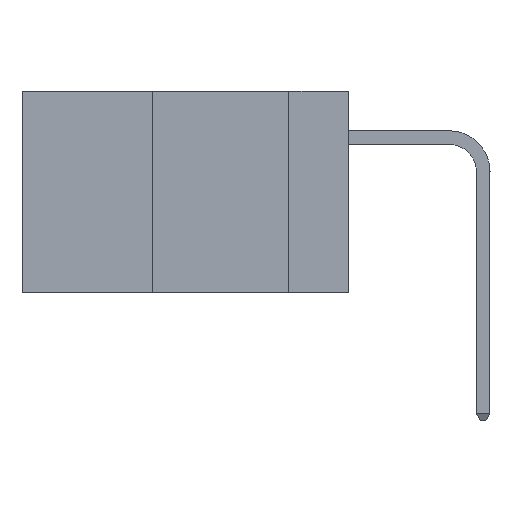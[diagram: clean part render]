
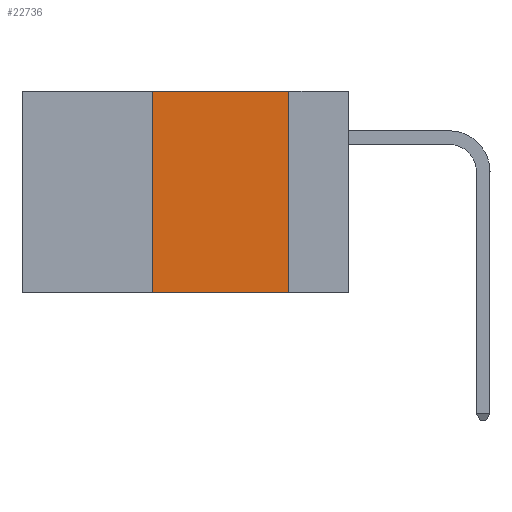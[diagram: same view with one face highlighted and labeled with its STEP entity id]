
A CAD part, left-side view. The second image highlights one B-rep face of the part: STEP entity #22736.
In plain terms, the highlighted planar face has unit normal (-1, 0, 0).
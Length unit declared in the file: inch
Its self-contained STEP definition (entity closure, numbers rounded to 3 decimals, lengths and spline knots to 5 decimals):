
#1048 = CARTESIAN_POINT ( 'NONE',  ( 0., 0.11, 0. ) ) ;
#1820 = VERTEX_POINT ( 'NONE', #23831 ) ;
#2241 = VECTOR ( 'NONE', #38119, 39.37008 ) ;
#2506 = CARTESIAN_POINT ( 'NONE',  ( 0., 0.36, 0. ) ) ;
#2942 = DIRECTION ( 'NONE',  ( 0., 0., -1. ) ) ;
#4873 = LINE ( 'NONE', #1048, #40593 ) ;
#5224 = CARTESIAN_POINT ( 'NONE',  ( 0., 0.11, 0. ) ) ;
#9188 = VERTEX_POINT ( 'NONE', #5224 ) ;
#13684 = AXIS2_PLACEMENT_3D ( 'NONE', #34231, #21785, #2942 ) ;
#16561 = DIRECTION ( 'NONE',  ( 0., 0., -1. ) ) ;
#17226 = EDGE_CURVE ( 'NONE', #38704, #1820, #28112, .T. ) ;
#17746 = ORIENTED_EDGE ( 'NONE', *, *, #17226, .F. ) ;
#18509 = VERTEX_POINT ( 'NONE', #34358 ) ;
#19070 = LINE ( 'NONE', #28050, #2241 ) ;
#21109 = EDGE_CURVE ( 'NONE', #9188, #18509, #4873, .T. ) ;
#21785 = DIRECTION ( 'NONE',  ( 1., 0., 0. ) ) ;
#22375 = EDGE_CURVE ( 'NONE', #38704, #18509, #19070, .T. ) ;
#22736 = ADVANCED_FACE ( 'NONE', ( #35819 ), #33830, .F. ) ;
#23115 = EDGE_CURVE ( 'NONE', #1820, #9188, #33341, .T. ) ;
#23831 = CARTESIAN_POINT ( 'NONE',  ( 0., 0.36, 0. ) ) ;
#25270 = EDGE_LOOP ( 'NONE', ( #32203, #31920, #17746, #28248 ) ) ;
#27684 = DIRECTION ( 'NONE',  ( 0., 0., 1. ) ) ;
#28050 = CARTESIAN_POINT ( 'NONE',  ( 0., 0.6, -0.37 ) ) ;
#28112 = LINE ( 'NONE', #2506, #31997 ) ;
#28248 = ORIENTED_EDGE ( 'NONE', *, *, #22375, .T. ) ;
#30471 = CARTESIAN_POINT ( 'NONE',  ( 0., 0.36, -0.37 ) ) ;
#31192 = DIRECTION ( 'NONE',  ( 0., -1., 0. ) ) ;
#31920 = ORIENTED_EDGE ( 'NONE', *, *, #23115, .F. ) ;
#31997 = VECTOR ( 'NONE', #27684, 39.37008 ) ;
#32203 = ORIENTED_EDGE ( 'NONE', *, *, #21109, .F. ) ;
#33341 = LINE ( 'NONE', #37854, #40813 ) ;
#33830 = PLANE ( 'NONE',  #13684 ) ;
#34231 = CARTESIAN_POINT ( 'NONE',  ( 0., 0.6, 0. ) ) ;
#34358 = CARTESIAN_POINT ( 'NONE',  ( 0., 0.11, -0.37 ) ) ;
#35819 = FACE_OUTER_BOUND ( 'NONE', #25270, .T. ) ;
#37854 = CARTESIAN_POINT ( 'NONE',  ( 0., 0.6, 0. ) ) ;
#38119 = DIRECTION ( 'NONE',  ( 0., -1., 0. ) ) ;
#38704 = VERTEX_POINT ( 'NONE', #30471 ) ;
#40593 = VECTOR ( 'NONE', #16561, 39.37008 ) ;
#40813 = VECTOR ( 'NONE', #31192, 39.37008 ) ;
